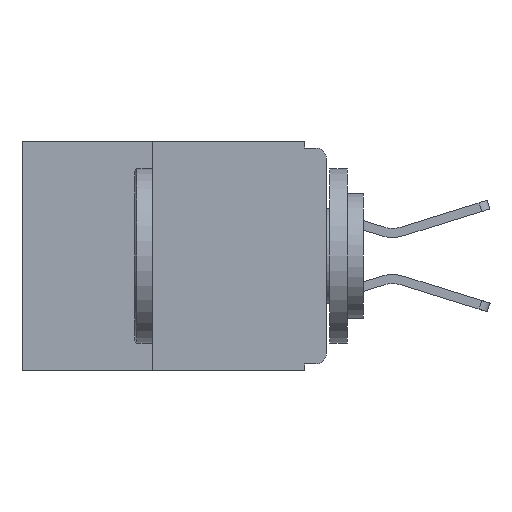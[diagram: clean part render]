
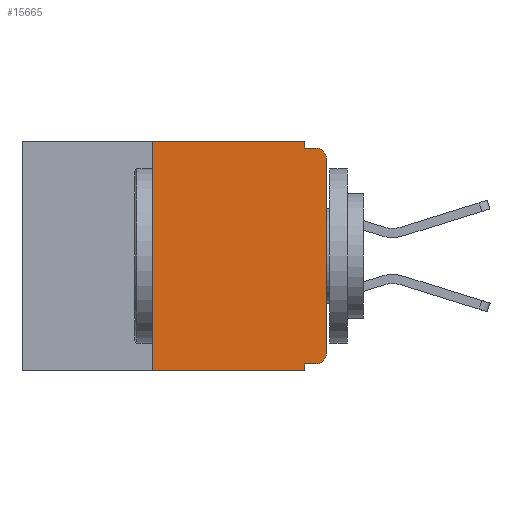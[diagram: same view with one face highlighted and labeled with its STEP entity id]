
A CAD part, left-side view. The second image highlights one B-rep face of the part: STEP entity #15665.
In plain terms, the highlighted planar face has unit normal (-1, 0, 0).
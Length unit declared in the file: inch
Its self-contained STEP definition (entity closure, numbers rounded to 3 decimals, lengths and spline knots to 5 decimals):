
#53 = DIRECTION ( 'NONE',  ( -1., 0., 0. ) ) ;
#131 = CARTESIAN_POINT ( 'NONE',  ( 0., 0., 0. ) ) ;
#360 = LINE ( 'NONE', #2939, #6762 ) ;
#569 = CIRCLE ( 'NONE', #5366, 0.015 ) ;
#1062 = CARTESIAN_POINT ( 'NONE',  ( 0., 0.015, -0.025 ) ) ;
#1063 = LINE ( 'NONE', #14272, #12260 ) ;
#1078 = EDGE_CURVE ( 'NONE', #14622, #12840, #569, .T. ) ;
#1174 = EDGE_CURVE ( 'NONE', #15727, #12780, #17526, .T. ) ;
#1179 = VECTOR ( 'NONE', #8401, 39.37008 ) ;
#1455 = CARTESIAN_POINT ( 'NONE',  ( 0., 0.031, -0.01 ) ) ;
#1486 = VERTEX_POINT ( 'NONE', #15187 ) ;
#1507 = CARTESIAN_POINT ( 'NONE',  ( 0., 0.25, -0.33 ) ) ;
#1543 = EDGE_CURVE ( 'NONE', #5657, #17705, #16441, .T. ) ;
#1944 = DIRECTION ( 'NONE',  ( 0., 0., -1. ) ) ;
#2109 = FACE_OUTER_BOUND ( 'NONE', #2340, .T. ) ;
#2214 = VERTEX_POINT ( 'NONE', #13206 ) ;
#2340 = EDGE_LOOP ( 'NONE', ( #3176, #7570, #5284, #8047, #6879, #11897, #2553, #17232, #4641, #13743 ) ) ;
#2452 = DIRECTION ( 'NONE',  ( 0., 0., -1. ) ) ;
#2553 = ORIENTED_EDGE ( 'NONE', *, *, #11600, .T. ) ;
#2569 = CARTESIAN_POINT ( 'NONE',  ( 0., 0.031, -0.33 ) ) ;
#2652 = DIRECTION ( 'NONE',  ( 0., -1., 0. ) ) ;
#2939 = CARTESIAN_POINT ( 'NONE',  ( 0., 0.031, -0.33 ) ) ;
#3054 = CARTESIAN_POINT ( 'NONE',  ( 0., 0.015, -0.01 ) ) ;
#3176 = ORIENTED_EDGE ( 'NONE', *, *, #14116, .T. ) ;
#3493 = CARTESIAN_POINT ( 'NONE',  ( 0., 0.031, 0. ) ) ;
#3735 = VERTEX_POINT ( 'NONE', #2569 ) ;
#3879 = EDGE_CURVE ( 'NONE', #5657, #14616, #9619, .T. ) ;
#4477 = CARTESIAN_POINT ( 'NONE',  ( 0., 0.015, -0.32 ) ) ;
#4641 = ORIENTED_EDGE ( 'NONE', *, *, #1543, .F. ) ;
#4903 = CARTESIAN_POINT ( 'NONE',  ( 0., 0.437, 0. ) ) ;
#5284 = ORIENTED_EDGE ( 'NONE', *, *, #13271, .F. ) ;
#5366 = AXIS2_PLACEMENT_3D ( 'NONE', #1062, #10053, #2452 ) ;
#5657 = VERTEX_POINT ( 'NONE', #4477 ) ;
#5838 = LINE ( 'NONE', #131, #13104 ) ;
#5864 = CARTESIAN_POINT ( 'NONE',  ( 0., 0., -0.025 ) ) ;
#5902 = DIRECTION ( 'NONE',  ( 0., 0., 1. ) ) ;
#6563 = CARTESIAN_POINT ( 'NONE',  ( 0., 0.031, 0. ) ) ;
#6609 = DIRECTION ( 'NONE',  ( 0., 0., -1. ) ) ;
#6762 = VECTOR ( 'NONE', #10231, 39.37008 ) ;
#6879 = ORIENTED_EDGE ( 'NONE', *, *, #15669, .F. ) ;
#7570 = ORIENTED_EDGE ( 'NONE', *, *, #1078, .T. ) ;
#8020 = VECTOR ( 'NONE', #5902, 39.37008 ) ;
#8047 = ORIENTED_EDGE ( 'NONE', *, *, #1174, .F. ) ;
#8401 = DIRECTION ( 'NONE',  ( 0., -1., 0. ) ) ;
#8523 = CARTESIAN_POINT ( 'NONE',  ( 0., 0.437, -0.33 ) ) ;
#8781 = CARTESIAN_POINT ( 'NONE',  ( 0., 0., -0.305 ) ) ;
#9247 = CARTESIAN_POINT ( 'NONE',  ( 0., 0.437, 0. ) ) ;
#9517 = AXIS2_PLACEMENT_3D ( 'NONE', #9247, #12085, #1944 ) ;
#9619 = CIRCLE ( 'NONE', #17197, 0.015 ) ;
#9722 = DIRECTION ( 'NONE',  ( 0., 0., -1. ) ) ;
#10053 = DIRECTION ( 'NONE',  ( -1., 0., 0. ) ) ;
#10231 = DIRECTION ( 'NONE',  ( 0., 0., -1. ) ) ;
#10687 = PLANE ( 'NONE',  #9517 ) ;
#11200 = CARTESIAN_POINT ( 'NONE',  ( 0., 0.031, -0.32 ) ) ;
#11600 = EDGE_CURVE ( 'NONE', #1486, #3735, #16588, .T. ) ;
#11605 = DIRECTION ( 'NONE',  ( 0., 1., 0. ) ) ;
#11897 = ORIENTED_EDGE ( 'NONE', *, *, #18100, .F. ) ;
#12085 = DIRECTION ( 'NONE',  ( 1., 0., 0. ) ) ;
#12260 = VECTOR ( 'NONE', #2652, 39.37008 ) ;
#12321 = LINE ( 'NONE', #1507, #8020 ) ;
#12780 = VERTEX_POINT ( 'NONE', #1455 ) ;
#12840 = VERTEX_POINT ( 'NONE', #3054 ) ;
#13104 = VECTOR ( 'NONE', #18639, 39.37008 ) ;
#13206 = CARTESIAN_POINT ( 'NONE',  ( 0., 0.25, 0. ) ) ;
#13271 = EDGE_CURVE ( 'NONE', #12780, #12840, #1063, .T. ) ;
#13743 = ORIENTED_EDGE ( 'NONE', *, *, #3879, .T. ) ;
#13798 = VECTOR ( 'NONE', #6609, 39.37008 ) ;
#14063 = EDGE_CURVE ( 'NONE', #17705, #3735, #360, .T. ) ;
#14116 = EDGE_CURVE ( 'NONE', #14616, #14622, #5838, .T. ) ;
#14272 = CARTESIAN_POINT ( 'NONE',  ( 0., 0., -0.01 ) ) ;
#14616 = VERTEX_POINT ( 'NONE', #8781 ) ;
#14622 = VERTEX_POINT ( 'NONE', #5864 ) ;
#14997 = CARTESIAN_POINT ( 'NONE',  ( 0., 0.015, -0.305 ) ) ;
#15008 = DIRECTION ( 'NONE',  ( 0., -1., 0. ) ) ;
#15095 = VECTOR ( 'NONE', #11605, 39.37008 ) ;
#15187 = CARTESIAN_POINT ( 'NONE',  ( 0., 0.25, -0.33 ) ) ;
#15587 = CARTESIAN_POINT ( 'NONE',  ( 0., 0., -0.32 ) ) ;
#15665 = ADVANCED_FACE ( 'NONE', ( #2109 ), #10687, .F. ) ;
#15669 = EDGE_CURVE ( 'NONE', #2214, #15727, #17024, .T. ) ;
#15727 = VERTEX_POINT ( 'NONE', #3493 ) ;
#16441 = LINE ( 'NONE', #15587, #15095 ) ;
#16588 = LINE ( 'NONE', #8523, #1179 ) ;
#17024 = LINE ( 'NONE', #4903, #17463 ) ;
#17197 = AXIS2_PLACEMENT_3D ( 'NONE', #14997, #53, #9722 ) ;
#17232 = ORIENTED_EDGE ( 'NONE', *, *, #14063, .F. ) ;
#17463 = VECTOR ( 'NONE', #15008, 39.37008 ) ;
#17526 = LINE ( 'NONE', #6563, #13798 ) ;
#17705 = VERTEX_POINT ( 'NONE', #11200 ) ;
#18100 = EDGE_CURVE ( 'NONE', #1486, #2214, #12321, .T. ) ;
#18639 = DIRECTION ( 'NONE',  ( 0., 0., 1. ) ) ;
